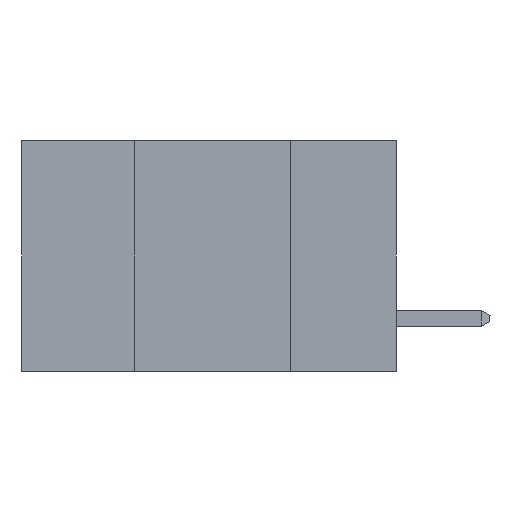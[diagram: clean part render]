
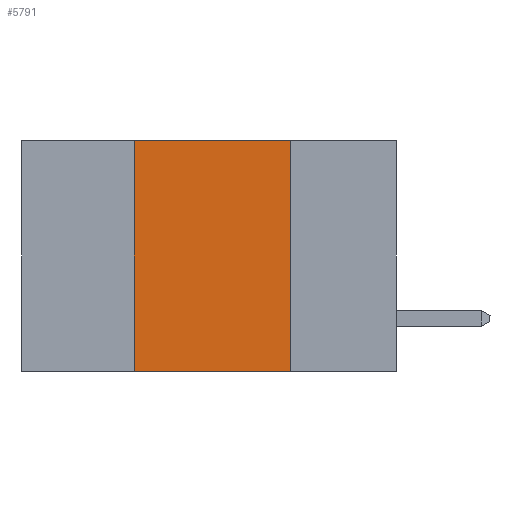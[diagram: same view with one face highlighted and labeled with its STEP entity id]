
A CAD part, left-side view. The second image highlights one B-rep face of the part: STEP entity #5791.
In plain terms, the highlighted planar face has unit normal (-1, 0, 0).
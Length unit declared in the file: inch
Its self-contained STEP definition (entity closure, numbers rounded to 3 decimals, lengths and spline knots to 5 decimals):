
#498 = CARTESIAN_POINT ( 'NONE',  ( 0., 0.42, 0. ) ) ;
#621 = VECTOR ( 'NONE', #3149, 39.37008 ) ;
#1223 = CARTESIAN_POINT ( 'NONE',  ( 0., 0.17, -0.37 ) ) ;
#1320 = VERTEX_POINT ( 'NONE', #498 ) ;
#1434 = FACE_OUTER_BOUND ( 'NONE', #2601, .T. ) ;
#2432 = CARTESIAN_POINT ( 'NONE',  ( 0., 0.17, -0.37 ) ) ;
#2516 = CARTESIAN_POINT ( 'NONE',  ( 0., 0.17, 0. ) ) ;
#2601 = EDGE_LOOP ( 'NONE', ( #7565, #4258, #12277, #12035 ) ) ;
#2909 = DIRECTION ( 'NONE',  ( 0., 0., 1. ) ) ;
#3149 = DIRECTION ( 'NONE',  ( 0., -1., 0. ) ) ;
#3520 = VECTOR ( 'NONE', #13572, 39.37008 ) ;
#3846 = AXIS2_PLACEMENT_3D ( 'NONE', #4817, #13940, #6121 ) ;
#4258 = ORIENTED_EDGE ( 'NONE', *, *, #5015, .F. ) ;
#4817 = CARTESIAN_POINT ( 'NONE',  ( 0., 0.6, 0. ) ) ;
#5015 = EDGE_CURVE ( 'NONE', #1320, #7929, #7703, .T. ) ;
#5126 = CARTESIAN_POINT ( 'NONE',  ( 0., 0.42, -0.37 ) ) ;
#5134 = DIRECTION ( 'NONE',  ( 0., 0., -1. ) ) ;
#5791 = ADVANCED_FACE ( 'NONE', ( #1434 ), #10001, .F. ) ;
#6041 = VERTEX_POINT ( 'NONE', #1223 ) ;
#6121 = DIRECTION ( 'NONE',  ( 0., 0., -1. ) ) ;
#6978 = LINE ( 'NONE', #2432, #13520 ) ;
#7565 = ORIENTED_EDGE ( 'NONE', *, *, #8529, .F. ) ;
#7703 = LINE ( 'NONE', #12319, #621 ) ;
#7929 = VERTEX_POINT ( 'NONE', #2516 ) ;
#7985 = LINE ( 'NONE', #9447, #14466 ) ;
#8529 = EDGE_CURVE ( 'NONE', #7929, #6041, #6978, .T. ) ;
#9378 = EDGE_CURVE ( 'NONE', #10932, #6041, #13564, .T. ) ;
#9447 = CARTESIAN_POINT ( 'NONE',  ( 0., 0.42, -0.37 ) ) ;
#10001 = PLANE ( 'NONE',  #3846 ) ;
#10932 = VERTEX_POINT ( 'NONE', #5126 ) ;
#11147 = EDGE_CURVE ( 'NONE', #10932, #1320, #7985, .T. ) ;
#12035 = ORIENTED_EDGE ( 'NONE', *, *, #9378, .T. ) ;
#12253 = CARTESIAN_POINT ( 'NONE',  ( 0., 0.6, -0.37 ) ) ;
#12277 = ORIENTED_EDGE ( 'NONE', *, *, #11147, .F. ) ;
#12319 = CARTESIAN_POINT ( 'NONE',  ( 0., 0.6, 0. ) ) ;
#13520 = VECTOR ( 'NONE', #5134, 39.37008 ) ;
#13564 = LINE ( 'NONE', #12253, #3520 ) ;
#13572 = DIRECTION ( 'NONE',  ( 0., -1., 0. ) ) ;
#13940 = DIRECTION ( 'NONE',  ( 1., 0., 0. ) ) ;
#14466 = VECTOR ( 'NONE', #2909, 39.37008 ) ;
